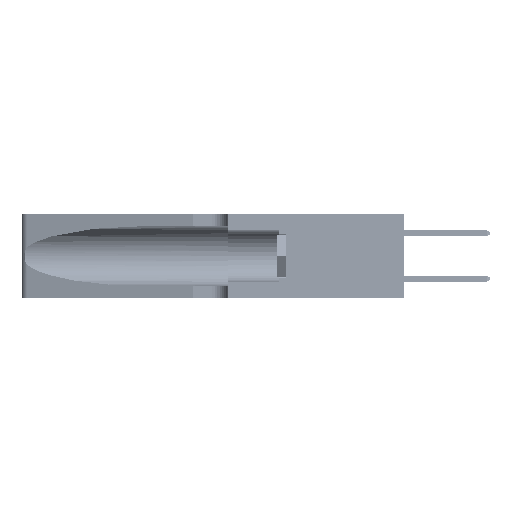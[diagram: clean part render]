
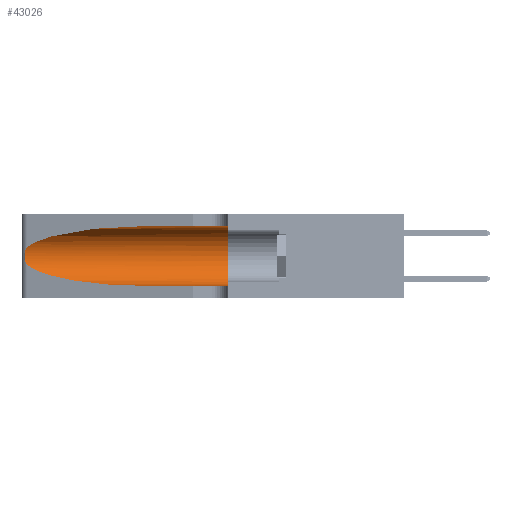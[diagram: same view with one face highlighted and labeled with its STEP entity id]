
A CAD part, left-side view. The second image highlights one B-rep face of the part: STEP entity #43026.
In plain terms, the highlighted cylindrical face has radius 3.308 mm (diameter 6.617 mm), a partial arc.
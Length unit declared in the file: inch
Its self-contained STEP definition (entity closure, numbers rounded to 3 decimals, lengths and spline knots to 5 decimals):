
#862 = VERTEX_POINT ( 'NONE', #26330 ) ;
#1255 = CARTESIAN_POINT ( 'NONE',  ( 0.26075, 1.23896, 0.19203 ) ) ;
#1555 = VERTEX_POINT ( 'NONE', #22923 ) ;
#2008 = DIRECTION ( 'NONE',  ( 0., 0., -1. ) ) ;
#3486 = EDGE_CURVE ( 'NONE', #1555, #29440, #39562, .T. ) ;
#4245 = CARTESIAN_POINT ( 'NONE',  ( 0.26017, 1.23833, 0.17102 ) ) ;
#6702 = EDGE_CURVE ( 'NONE', #25349, #33815, #29855, .T. ) ;
#7191 = DIRECTION ( 'NONE',  ( 0., -1., 0. ) ) ;
#7549 = CARTESIAN_POINT ( 'NONE',  ( 0.2373, 1.15595, 0.28018 ) ) ;
#8264 = CARTESIAN_POINT ( 'NONE',  ( 0.25487, 1.22718, 0.22369 ) ) ;
#8449 = CARTESIAN_POINT ( 'NONE',  ( 0.25789, 1.23486, 0.15765 ) ) ;
#11563 = CARTESIAN_POINT ( 'NONE',  ( 0.1305, 0.72297, 0.31525 ) ) ;
#11750 = CARTESIAN_POINT ( 'NONE',  ( 0.25487, 1.22718, 0.22369 ) ) ;
#12647 = CARTESIAN_POINT ( 'NONE',  ( 0.25555, 1.22993, 0.14849 ) ) ;
#13665 = ORIENTED_EDGE ( 'NONE', *, *, #32339, .F. ) ;
#13715 = ORIENTED_EDGE ( 'NONE', *, *, #43974, .T. ) ;
#14535 = ORIENTED_EDGE ( 'NONE', *, *, #28678, .F. ) ;
#17097 = CARTESIAN_POINT ( 'NONE',  ( 0.1305, 1.61858, 0.05475 ) ) ;
#18084 = ORIENTED_EDGE ( 'NONE', *, *, #3486, .T. ) ;
#18156 = CARTESIAN_POINT ( 'NONE',  ( 0.1305, 0.72297, 0.05475 ) ) ;
#18635 = DIRECTION ( 'NONE',  ( 0., -1., 0. ) ) ;
#19539 = LINE ( 'NONE', #17097, #40491 ) ;
#19622 = CARTESIAN_POINT ( 'NONE',  ( 0.1305, 1.61858, 0.31525 ) ) ;
#20899 = CARTESIAN_POINT ( 'NONE',  ( 0.25787, 1.23484, 0.2124 ) ) ;
#21548 = CYLINDRICAL_SURFACE ( 'NONE', #46967, 0.13025 ) ;
#22923 = CARTESIAN_POINT ( 'NONE',  ( 0.25487, 1.22718, 0.14631 ) ) ;
#23231 = EDGE_CURVE ( 'NONE', #33815, #1555, #45244, .T. ) ;
#23601 = LINE ( 'NONE', #19622, #44557 ) ;
#24219 = CARTESIAN_POINT ( 'NONE',  ( 0.1305, 0.35, 0.185 ) ) ;
#24572 = CIRCLE ( 'NONE', #47406, 0.13025 ) ;
#25080 = CARTESIAN_POINT ( 'NONE',  ( 0.26018, 1.23835, 0.19895 ) ) ;
#25349 = VERTEX_POINT ( 'NONE', #51528 ) ;
#26330 = CARTESIAN_POINT ( 'NONE',  ( 0.1305, 0.35, 0.31525 ) ) ;
#27088 = CARTESIAN_POINT ( 'NONE',  ( 0.1305, 1.61858, 0.185 ) ) ;
#28452 = DIRECTION ( 'NONE',  ( 0., 0., 1. ) ) ;
#28678 = EDGE_CURVE ( 'NONE', #25349, #862, #23601, .T. ) ;
#29325 = CARTESIAN_POINT ( 'NONE',  ( 0.26075, 1.23896, 0.178 ) ) ;
#29440 = VERTEX_POINT ( 'NONE', #31282 ) ;
#29855 =( BOUNDED_CURVE ( )  B_SPLINE_CURVE ( 3, ( #11563, #53363, #7549, #11750 ),
 .UNSPECIFIED., .F., .T. ) 
 B_SPLINE_CURVE_WITH_KNOTS ( ( 4, 4 ),
 ( 1.5708, 2.84003 ),
 .UNSPECIFIED. ) 
 CURVE ( )  GEOMETRIC_REPRESENTATION_ITEM ( )  RATIONAL_B_SPLINE_CURVE ( ( 1., 0.87, 0.87, 1. ) ) 
 REPRESENTATION_ITEM ( '' )  );
#31282 = CARTESIAN_POINT ( 'NONE',  ( 0.1305, 0.72297, 0.05475 ) ) ;
#32339 = EDGE_CURVE ( 'NONE', #862, #48852, #24572, .T. ) ;
#33102 = ORIENTED_EDGE ( 'NONE', *, *, #23231, .T. ) ;
#33343 = CARTESIAN_POINT ( 'NONE',  ( 0.25555, 1.22994, 0.2215 ) ) ;
#33521 = CARTESIAN_POINT ( 'NONE',  ( 0.25856, 1.23593, 0.16098 ) ) ;
#33815 = VERTEX_POINT ( 'NONE', #49288 ) ;
#34842 = CARTESIAN_POINT ( 'NONE',  ( 0.25487, 1.22718, 0.14631 ) ) ;
#37462 = EDGE_LOOP ( 'NONE', ( #38968, #33102, #18084, #13715, #13665, #14535 ) ) ;
#37699 = CARTESIAN_POINT ( 'NONE',  ( 0.25639, 1.23186, 0.15144 ) ) ;
#38968 = ORIENTED_EDGE ( 'NONE', *, *, #6702, .T. ) ;
#39199 = CARTESIAN_POINT ( 'NONE',  ( 0.1305, 0.35, 0.05475 ) ) ;
#39562 =( BOUNDED_CURVE ( )  B_SPLINE_CURVE ( 3, ( #34842, #47239, #43236, #18156 ),
 .UNSPECIFIED., .F., .F. ) 
 B_SPLINE_CURVE_WITH_KNOTS ( ( 4, 4 ),
 ( 3.44316, 4.71239 ),
 .UNSPECIFIED. ) 
 CURVE ( )  GEOMETRIC_REPRESENTATION_ITEM ( )  RATIONAL_B_SPLINE_CURVE ( ( 1., 0.87, 0.87, 1. ) ) 
 REPRESENTATION_ITEM ( '' )  );
#40491 = VECTOR ( 'NONE', #46357, 39.37008 ) ;
#41925 = CARTESIAN_POINT ( 'NONE',  ( 0.25487, 1.22718, 0.14631 ) ) ;
#43026 = ADVANCED_FACE ( 'NONE', ( #43784 ), #21548, .F. ) ;
#43236 = CARTESIAN_POINT ( 'NONE',  ( 0.18966, 0.96281, 0.05475 ) ) ;
#43784 = FACE_OUTER_BOUND ( 'NONE', #37462, .T. ) ;
#43974 = EDGE_CURVE ( 'NONE', #29440, #48852, #19539, .T. ) ;
#44557 = VECTOR ( 'NONE', #7191, 39.37008 ) ;
#45244 = B_SPLINE_CURVE_WITH_KNOTS ( 'NONE', 3,
 ( #8264, #33343, #45913, #20899, #50119, #25080, #1255, #29325, #4245, #33521, #8449, #37699, #12647, #41925 ),
 .UNSPECIFIED., .F., .F.,
 ( 4, 2, 2, 2, 2, 2, 4 ),
 ( 0., 0.00027, 0.00053, 0.00107, 0.0016, 0.00187, 0.00214 ),
 .UNSPECIFIED. ) ;
#45913 = CARTESIAN_POINT ( 'NONE',  ( 0.25639, 1.23184, 0.21858 ) ) ;
#46357 = DIRECTION ( 'NONE',  ( 0., -1., 0. ) ) ;
#46967 = AXIS2_PLACEMENT_3D ( 'NONE', #27088, #18635, #2008 ) ;
#47239 = CARTESIAN_POINT ( 'NONE',  ( 0.2373, 1.15595, 0.08982 ) ) ;
#47406 = AXIS2_PLACEMENT_3D ( 'NONE', #24219, #53421, #28452 ) ;
#48852 = VERTEX_POINT ( 'NONE', #39199 ) ;
#49288 = CARTESIAN_POINT ( 'NONE',  ( 0.25487, 1.22718, 0.22369 ) ) ;
#50119 = CARTESIAN_POINT ( 'NONE',  ( 0.25854, 1.2359, 0.20912 ) ) ;
#51528 = CARTESIAN_POINT ( 'NONE',  ( 0.1305, 0.72297, 0.31525 ) ) ;
#53363 = CARTESIAN_POINT ( 'NONE',  ( 0.18966, 0.96281, 0.31525 ) ) ;
#53421 = DIRECTION ( 'NONE',  ( 0., 1., 0. ) ) ;
